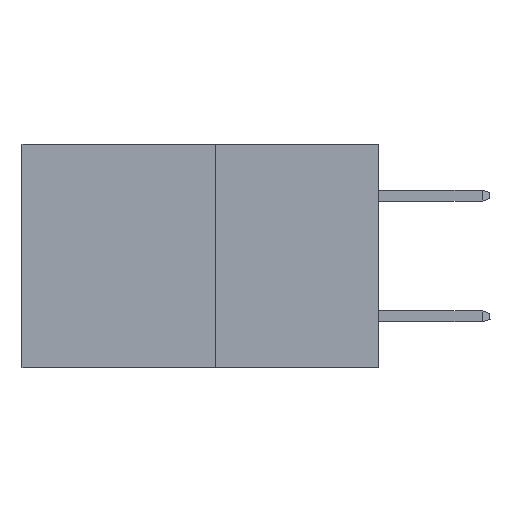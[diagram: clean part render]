
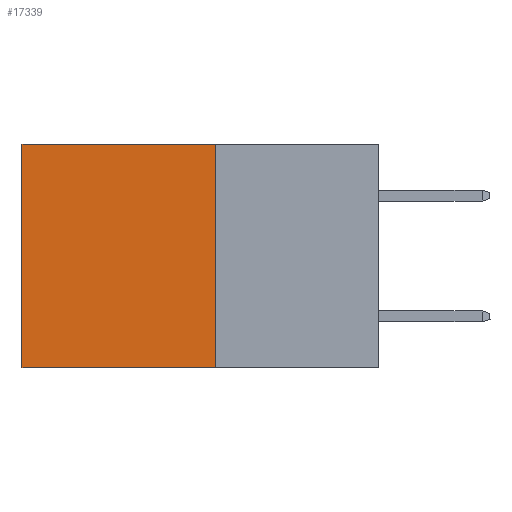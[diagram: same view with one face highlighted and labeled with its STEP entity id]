
A CAD part, left-side view. The second image highlights one B-rep face of the part: STEP entity #17339.
In plain terms, the highlighted planar face has unit normal (-1, 0, 0).
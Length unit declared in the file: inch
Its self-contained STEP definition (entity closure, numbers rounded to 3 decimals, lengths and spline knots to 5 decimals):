
#394 = EDGE_LOOP ( 'NONE', ( #5317, #20825, #19878, #4098 ) ) ;
#4098 = ORIENTED_EDGE ( 'NONE', *, *, #15039, .T. ) ;
#5109 = EDGE_CURVE ( 'NONE', #15436, #13618, #19709, .T. ) ;
#5228 = CARTESIAN_POINT ( 'NONE',  ( 0.277, 0.27, 0. ) ) ;
#5317 = ORIENTED_EDGE ( 'NONE', *, *, #5109, .T. ) ;
#5404 = DIRECTION ( 'NONE',  ( 0., 1., 0. ) ) ;
#5667 = CARTESIAN_POINT ( 'NONE',  ( 0.277, 0.27, -0.37 ) ) ;
#6144 = VERTEX_POINT ( 'NONE', #13970 ) ;
#8001 = CARTESIAN_POINT ( 'NONE',  ( 0.277, 0.59, -0.37 ) ) ;
#8156 = CARTESIAN_POINT ( 'NONE',  ( 0.277, 0.59, 0. ) ) ;
#9467 = VECTOR ( 'NONE', #5404, 39.37008 ) ;
#9736 = LINE ( 'NONE', #13305, #19158 ) ;
#10849 = EDGE_CURVE ( 'NONE', #6144, #13618, #24201, .T. ) ;
#11345 = VECTOR ( 'NONE', #19159, 39.37008 ) ;
#11581 = AXIS2_PLACEMENT_3D ( 'NONE', #23659, #11763, #25702 ) ;
#11763 = DIRECTION ( 'NONE',  ( 1., 0., 0. ) ) ;
#13305 = CARTESIAN_POINT ( 'NONE',  ( 0.277, 0.27, -0.37 ) ) ;
#13618 = VERTEX_POINT ( 'NONE', #8001 ) ;
#13970 = CARTESIAN_POINT ( 'NONE',  ( 0.277, 0.27, -0.37 ) ) ;
#14628 = VERTEX_POINT ( 'NONE', #5228 ) ;
#15039 = EDGE_CURVE ( 'NONE', #14628, #15436, #17913, .T. ) ;
#15436 = VERTEX_POINT ( 'NONE', #8156 ) ;
#15817 = EDGE_CURVE ( 'NONE', #14628, #6144, #9736, .T. ) ;
#17339 = ADVANCED_FACE ( 'NONE', ( #19369 ), #23753, .F. ) ;
#17913 = LINE ( 'NONE', #21180, #11345 ) ;
#19158 = VECTOR ( 'NONE', #25264, 39.37008 ) ;
#19159 = DIRECTION ( 'NONE',  ( 0., 1., 0. ) ) ;
#19369 = FACE_OUTER_BOUND ( 'NONE', #394, .T. ) ;
#19709 = LINE ( 'NONE', #20596, #24971 ) ;
#19878 = ORIENTED_EDGE ( 'NONE', *, *, #15817, .F. ) ;
#20596 = CARTESIAN_POINT ( 'NONE',  ( 0.277, 0.59, -0.37 ) ) ;
#20825 = ORIENTED_EDGE ( 'NONE', *, *, #10849, .F. ) ;
#21180 = CARTESIAN_POINT ( 'NONE',  ( 0.277, 0.27, 0. ) ) ;
#23608 = DIRECTION ( 'NONE',  ( 0., 0., -1. ) ) ;
#23659 = CARTESIAN_POINT ( 'NONE',  ( 0.277, 0.27, -0.37 ) ) ;
#23753 = PLANE ( 'NONE',  #11581 ) ;
#24201 = LINE ( 'NONE', #5667, #9467 ) ;
#24971 = VECTOR ( 'NONE', #23608, 39.37008 ) ;
#25264 = DIRECTION ( 'NONE',  ( 0., 0., -1. ) ) ;
#25702 = DIRECTION ( 'NONE',  ( 0., 0., -1. ) ) ;
